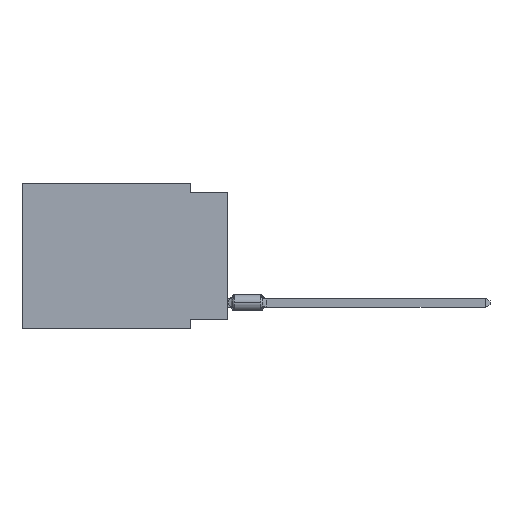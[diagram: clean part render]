
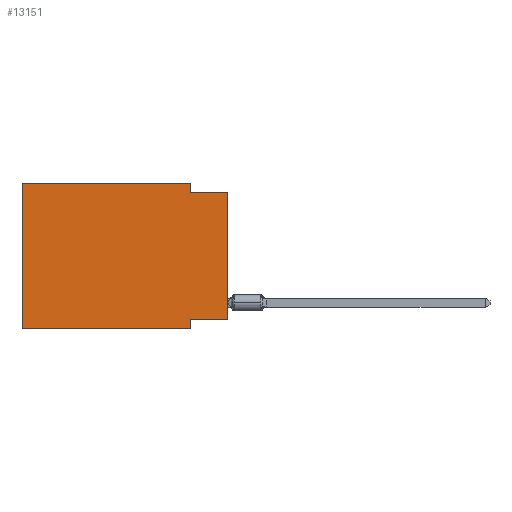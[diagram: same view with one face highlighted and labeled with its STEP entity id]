
A CAD part, left-side view. The second image highlights one B-rep face of the part: STEP entity #13151.
In plain terms, the highlighted planar face has unit normal (-1, 0, 0).
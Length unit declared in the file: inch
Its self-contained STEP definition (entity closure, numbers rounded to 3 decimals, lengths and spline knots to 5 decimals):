
#372 = DIRECTION ( 'NONE',  ( 0., 0., -1. ) ) ;
#714 = EDGE_LOOP ( 'NONE', ( #931, #18784, #17374, #23275, #20191, #14802, #4566, #16950 ) ) ;
#931 = ORIENTED_EDGE ( 'NONE', *, *, #14390, .T. ) ;
#966 = CARTESIAN_POINT ( 'NONE',  ( 0., 0.55, 0. ) ) ;
#1491 = CARTESIAN_POINT ( 'NONE',  ( 0., 0.55, -0.39 ) ) ;
#1590 = DIRECTION ( 'NONE',  ( 0., 0., -1. ) ) ;
#2405 = CARTESIAN_POINT ( 'NONE',  ( 0., 0.1, 0. ) ) ;
#3651 = DIRECTION ( 'NONE',  ( 0., -1., 0. ) ) ;
#3696 = CARTESIAN_POINT ( 'NONE',  ( 0., 0.55, 0. ) ) ;
#3828 = VECTOR ( 'NONE', #1590, 39.37008 ) ;
#4209 = VECTOR ( 'NONE', #3651, 39.37008 ) ;
#4566 = ORIENTED_EDGE ( 'NONE', *, *, #9570, .F. ) ;
#4573 = VECTOR ( 'NONE', #21809, 39.37008 ) ;
#5231 = CARTESIAN_POINT ( 'NONE',  ( 0., 0.1, -0.39 ) ) ;
#5621 = EDGE_CURVE ( 'NONE', #15821, #13782, #16477, .T. ) ;
#6535 = CARTESIAN_POINT ( 'NONE',  ( 0., 0., 0. ) ) ;
#7314 = DIRECTION ( 'NONE',  ( 0., 1., 0. ) ) ;
#8783 = VECTOR ( 'NONE', #14313, 39.37008 ) ;
#9169 = EDGE_CURVE ( 'NONE', #15821, #10658, #19296, .T. ) ;
#9570 = EDGE_CURVE ( 'NONE', #19267, #10658, #12918, .T. ) ;
#10022 = DIRECTION ( 'NONE',  ( 0., 0., -1. ) ) ;
#10084 = LINE ( 'NONE', #6535, #8783 ) ;
#10658 = VERTEX_POINT ( 'NONE', #5231 ) ;
#10974 = EDGE_CURVE ( 'NONE', #13018, #19267, #15591, .T. ) ;
#11198 = CARTESIAN_POINT ( 'NONE',  ( 0., 0., -0.365 ) ) ;
#11817 = PLANE ( 'NONE',  #14517 ) ;
#12083 = CARTESIAN_POINT ( 'NONE',  ( 0., 0.55, 0. ) ) ;
#12550 = EDGE_CURVE ( 'NONE', #13782, #20528, #18397, .T. ) ;
#12820 = CARTESIAN_POINT ( 'NONE',  ( 0., 0.1, -0.365 ) ) ;
#12857 = CARTESIAN_POINT ( 'NONE',  ( 0., 0., -0.025 ) ) ;
#12918 = LINE ( 'NONE', #20923, #3828 ) ;
#13018 = VERTEX_POINT ( 'NONE', #11198 ) ;
#13150 = EDGE_CURVE ( 'NONE', #20528, #21895, #15788, .T. ) ;
#13151 = ADVANCED_FACE ( 'NONE', ( #21866 ), #11817, .F. ) ;
#13782 = VERTEX_POINT ( 'NONE', #3696 ) ;
#14313 = DIRECTION ( 'NONE',  ( 0., 0., 1. ) ) ;
#14390 = EDGE_CURVE ( 'NONE', #13018, #19038, #10084, .T. ) ;
#14517 = AXIS2_PLACEMENT_3D ( 'NONE', #12083, #21743, #372 ) ;
#14802 = ORIENTED_EDGE ( 'NONE', *, *, #9169, .T. ) ;
#14870 = LINE ( 'NONE', #21076, #19471 ) ;
#15381 = CARTESIAN_POINT ( 'NONE',  ( 0., 0.1, 0. ) ) ;
#15591 = LINE ( 'NONE', #24842, #16470 ) ;
#15788 = LINE ( 'NONE', #2405, #23028 ) ;
#15821 = VERTEX_POINT ( 'NONE', #1491 ) ;
#16116 = VECTOR ( 'NONE', #24230, 39.37008 ) ;
#16470 = VECTOR ( 'NONE', #7314, 39.37008 ) ;
#16477 = LINE ( 'NONE', #24202, #4573 ) ;
#16774 = CARTESIAN_POINT ( 'NONE',  ( 0., 0.1, -0.025 ) ) ;
#16898 = CARTESIAN_POINT ( 'NONE',  ( 0., 0.55, -0.39 ) ) ;
#16950 = ORIENTED_EDGE ( 'NONE', *, *, #10974, .F. ) ;
#17374 = ORIENTED_EDGE ( 'NONE', *, *, #13150, .F. ) ;
#17833 = EDGE_CURVE ( 'NONE', #21895, #19038, #14870, .T. ) ;
#18397 = LINE ( 'NONE', #966, #16116 ) ;
#18784 = ORIENTED_EDGE ( 'NONE', *, *, #17833, .F. ) ;
#19038 = VERTEX_POINT ( 'NONE', #12857 ) ;
#19267 = VERTEX_POINT ( 'NONE', #12820 ) ;
#19296 = LINE ( 'NONE', #16898, #4209 ) ;
#19471 = VECTOR ( 'NONE', #24492, 39.37008 ) ;
#20191 = ORIENTED_EDGE ( 'NONE', *, *, #5621, .F. ) ;
#20528 = VERTEX_POINT ( 'NONE', #15381 ) ;
#20923 = CARTESIAN_POINT ( 'NONE',  ( 0., 0.1, -0.39 ) ) ;
#21076 = CARTESIAN_POINT ( 'NONE',  ( 0., 0., -0.025 ) ) ;
#21743 = DIRECTION ( 'NONE',  ( 1., 0., 0. ) ) ;
#21809 = DIRECTION ( 'NONE',  ( 0., 0., 1. ) ) ;
#21866 = FACE_OUTER_BOUND ( 'NONE', #714, .T. ) ;
#21895 = VERTEX_POINT ( 'NONE', #16774 ) ;
#23028 = VECTOR ( 'NONE', #10022, 39.37008 ) ;
#23275 = ORIENTED_EDGE ( 'NONE', *, *, #12550, .F. ) ;
#24202 = CARTESIAN_POINT ( 'NONE',  ( 0., 0.55, 0. ) ) ;
#24230 = DIRECTION ( 'NONE',  ( 0., -1., 0. ) ) ;
#24492 = DIRECTION ( 'NONE',  ( 0., -1., 0. ) ) ;
#24842 = CARTESIAN_POINT ( 'NONE',  ( 0., 0., -0.365 ) ) ;
